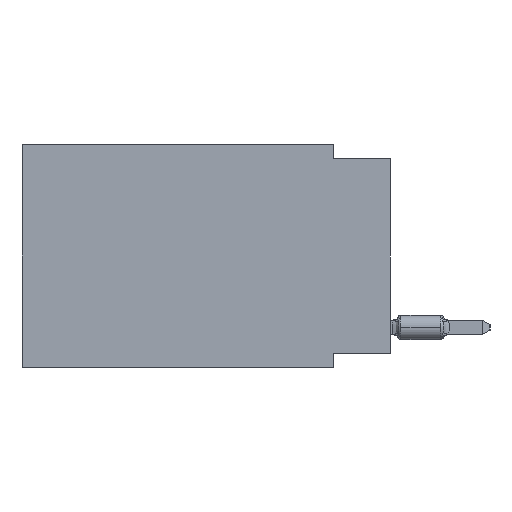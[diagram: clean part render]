
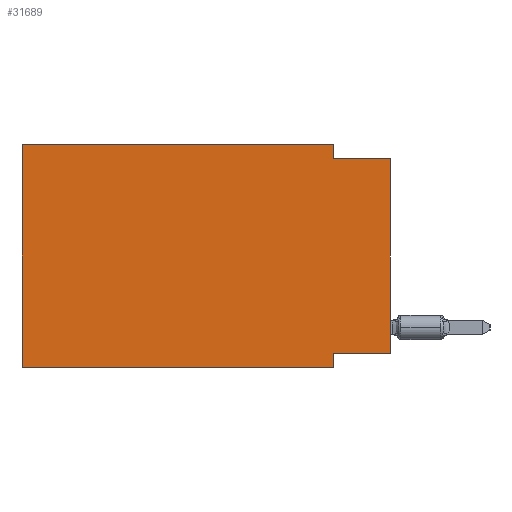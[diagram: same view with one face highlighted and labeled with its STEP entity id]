
A CAD part, left-side view. The second image highlights one B-rep face of the part: STEP entity #31689.
In plain terms, the highlighted planar face has unit normal (-1, 0, 0).
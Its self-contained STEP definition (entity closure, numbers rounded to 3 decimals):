
#799 = VECTOR ( 'NONE', #13900, 1000. ) ;
#1292 = CARTESIAN_POINT ( 'NONE',  ( 0., 2.54, -9.906 ) ) ;
#1494 = FACE_OUTER_BOUND ( 'NONE', #29748, .T. ) ;
#1999 = VECTOR ( 'NONE', #31112, 1000. ) ;
#5019 = ORIENTED_EDGE ( 'NONE', *, *, #18637, .F. ) ;
#5149 = ORIENTED_EDGE ( 'NONE', *, *, #52694, .F. ) ;
#5425 = VECTOR ( 'NONE', #44593, 1000. ) ;
#6045 = ORIENTED_EDGE ( 'NONE', *, *, #39098, .T. ) ;
#12735 = DIRECTION ( 'NONE',  ( 0., 0., 1. ) ) ;
#13085 = EDGE_CURVE ( 'NONE', #52170, #44683, #44007, .T. ) ;
#13900 = DIRECTION ( 'NONE',  ( 0., -1., 0. ) ) ;
#14649 = CARTESIAN_POINT ( 'NONE',  ( 0., 0., -9.271 ) ) ;
#15002 = ORIENTED_EDGE ( 'NONE', *, *, #31200, .F. ) ;
#17910 = DIRECTION ( 'NONE',  ( 0., 0., -1. ) ) ;
#18637 = EDGE_CURVE ( 'NONE', #56591, #40445, #44015, .T. ) ;
#18959 = PLANE ( 'NONE',  #36270 ) ;
#19694 = VERTEX_POINT ( 'NONE', #30187 ) ;
#22025 = CARTESIAN_POINT ( 'NONE',  ( 0., 0., -0.635 ) ) ;
#23740 = VERTEX_POINT ( 'NONE', #22025 ) ;
#24390 = CARTESIAN_POINT ( 'NONE',  ( 0., 0., -9.271 ) ) ;
#25507 = CARTESIAN_POINT ( 'NONE',  ( 0., 16.383, -9.906 ) ) ;
#28749 = CARTESIAN_POINT ( 'NONE',  ( 0., 0., -0.635 ) ) ;
#29748 = EDGE_LOOP ( 'NONE', ( #6045, #35300, #5019, #5149, #53862, #43433, #15002, #39025 ) ) ;
#30148 = VECTOR ( 'NONE', #37563, 1000. ) ;
#30187 = CARTESIAN_POINT ( 'NONE',  ( 0., 2.54, -9.906 ) ) ;
#30853 = LINE ( 'NONE', #31420, #5425 ) ;
#31112 = DIRECTION ( 'NONE',  ( 0., 0., 1. ) ) ;
#31200 = EDGE_CURVE ( 'NONE', #55113, #19694, #53958, .T. ) ;
#31420 = CARTESIAN_POINT ( 'NONE',  ( 0., 16.383, -9.906 ) ) ;
#31689 = ADVANCED_FACE ( 'NONE', ( #1494 ), #18959, .F. ) ;
#32430 = VERTEX_POINT ( 'NONE', #14649 ) ;
#33119 = EDGE_CURVE ( 'NONE', #40445, #23740, #46213, .T. ) ;
#34502 = LINE ( 'NONE', #42523, #54108 ) ;
#35284 = VECTOR ( 'NONE', #17910, 1000. ) ;
#35300 = ORIENTED_EDGE ( 'NONE', *, *, #33119, .F. ) ;
#35486 = VECTOR ( 'NONE', #54520, 1000. ) ;
#35954 = LINE ( 'NONE', #53120, #799 ) ;
#36270 = AXIS2_PLACEMENT_3D ( 'NONE', #36437, #53886, #46422 ) ;
#36437 = CARTESIAN_POINT ( 'NONE',  ( 0., 16.383, 0. ) ) ;
#36627 = EDGE_CURVE ( 'NONE', #32430, #55113, #45306, .T. ) ;
#37563 = DIRECTION ( 'NONE',  ( 0., 1., 0. ) ) ;
#37842 = CARTESIAN_POINT ( 'NONE',  ( 0., 16.383, 0. ) ) ;
#37859 = CARTESIAN_POINT ( 'NONE',  ( 0., 2.54, 0. ) ) ;
#39025 = ORIENTED_EDGE ( 'NONE', *, *, #36627, .F. ) ;
#39098 = EDGE_CURVE ( 'NONE', #32430, #23740, #34502, .T. ) ;
#39990 = CARTESIAN_POINT ( 'NONE',  ( 0., 16.383, 0. ) ) ;
#40283 = CARTESIAN_POINT ( 'NONE',  ( 0., 2.54, 0. ) ) ;
#40445 = VERTEX_POINT ( 'NONE', #52538 ) ;
#42523 = CARTESIAN_POINT ( 'NONE',  ( 0., 0., 0. ) ) ;
#43433 = ORIENTED_EDGE ( 'NONE', *, *, #48282, .T. ) ;
#44007 = LINE ( 'NONE', #39990, #1999 ) ;
#44015 = LINE ( 'NONE', #40283, #52554 ) ;
#44593 = DIRECTION ( 'NONE',  ( 0., -1., 0. ) ) ;
#44683 = VERTEX_POINT ( 'NONE', #37842 ) ;
#45306 = LINE ( 'NONE', #24390, #30148 ) ;
#46213 = LINE ( 'NONE', #28749, #35486 ) ;
#46422 = DIRECTION ( 'NONE',  ( 0., 0., -1. ) ) ;
#48282 = EDGE_CURVE ( 'NONE', #52170, #19694, #30853, .T. ) ;
#48478 = CARTESIAN_POINT ( 'NONE',  ( 0., 2.54, -9.271 ) ) ;
#52170 = VERTEX_POINT ( 'NONE', #25507 ) ;
#52538 = CARTESIAN_POINT ( 'NONE',  ( 0., 2.54, -0.635 ) ) ;
#52554 = VECTOR ( 'NONE', #53447, 1000. ) ;
#52694 = EDGE_CURVE ( 'NONE', #44683, #56591, #35954, .T. ) ;
#53120 = CARTESIAN_POINT ( 'NONE',  ( 0., 16.383, 0. ) ) ;
#53447 = DIRECTION ( 'NONE',  ( 0., 0., -1. ) ) ;
#53862 = ORIENTED_EDGE ( 'NONE', *, *, #13085, .F. ) ;
#53886 = DIRECTION ( 'NONE',  ( 1., 0., 0. ) ) ;
#53958 = LINE ( 'NONE', #1292, #35284 ) ;
#54108 = VECTOR ( 'NONE', #12735, 1000. ) ;
#54520 = DIRECTION ( 'NONE',  ( 0., -1., 0. ) ) ;
#55113 = VERTEX_POINT ( 'NONE', #48478 ) ;
#56591 = VERTEX_POINT ( 'NONE', #37859 ) ;
